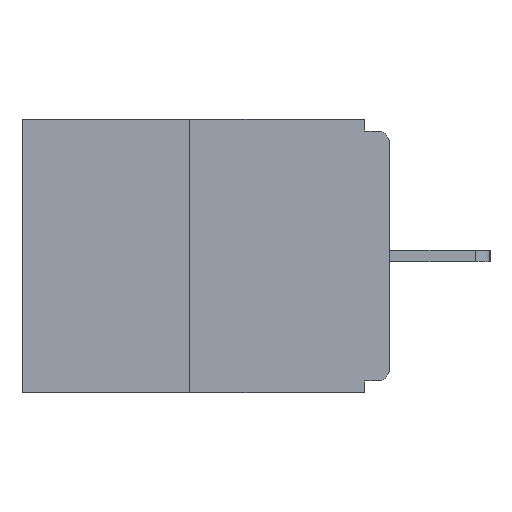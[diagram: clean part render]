
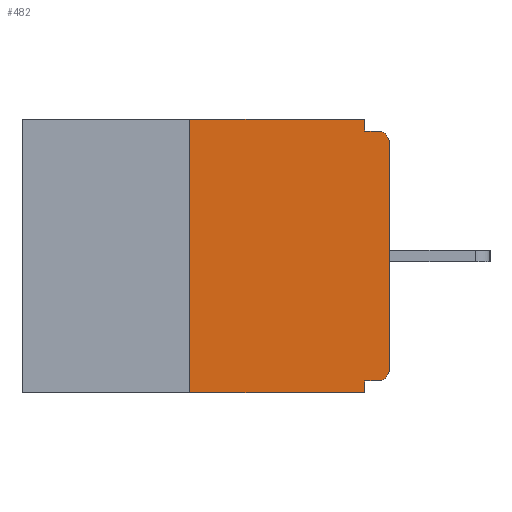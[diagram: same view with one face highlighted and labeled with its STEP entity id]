
A CAD part, left-side view. The second image highlights one B-rep face of the part: STEP entity #482.
In plain terms, the highlighted planar face has unit normal (-1, 0, 0).
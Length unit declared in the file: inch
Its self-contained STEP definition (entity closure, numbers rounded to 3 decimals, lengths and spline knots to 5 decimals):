
#51 = ORIENTED_EDGE ( 'NONE', *, *, #4367, .T. ) ;
#288 = DIRECTION ( 'NONE',  ( 0., 0., 1. ) ) ;
#311 = DIRECTION ( 'NONE',  ( -1., 0., 0. ) ) ;
#482 = ADVANCED_FACE ( 'NONE', ( #3917 ), #5129, .F. ) ;
#664 = AXIS2_PLACEMENT_3D ( 'NONE', #2507, #10840, #3674 ) ;
#820 = VERTEX_POINT ( 'NONE', #11308 ) ;
#857 = EDGE_CURVE ( 'NONE', #13726, #4578, #2613, .T. ) ;
#947 = VERTEX_POINT ( 'NONE', #15404 ) ;
#965 = EDGE_CURVE ( 'NONE', #13865, #2739, #7038, .T. ) ;
#1092 = AXIS2_PLACEMENT_3D ( 'NONE', #5073, #3951, #8962 ) ;
#1094 = VECTOR ( 'NONE', #6309, 39.37008 ) ;
#1556 = CARTESIAN_POINT ( 'NONE',  ( 0., 0., -0.328 ) ) ;
#1710 = EDGE_CURVE ( 'NONE', #14695, #947, #11724, .T. ) ;
#1881 = ORIENTED_EDGE ( 'NONE', *, *, #857, .T. ) ;
#1944 = ORIENTED_EDGE ( 'NONE', *, *, #12583, .F. ) ;
#2138 = DIRECTION ( 'NONE',  ( 0., 0., -1. ) ) ;
#2236 = VECTOR ( 'NONE', #12842, 39.37008 ) ;
#2246 = LINE ( 'NONE', #11869, #4642 ) ;
#2437 = CARTESIAN_POINT ( 'NONE',  ( 0., 0.031, -0.343 ) ) ;
#2507 = CARTESIAN_POINT ( 'NONE',  ( 0., 0.015, -0.313 ) ) ;
#2613 = LINE ( 'NONE', #5681, #2236 ) ;
#2739 = VERTEX_POINT ( 'NONE', #4199 ) ;
#3428 = VECTOR ( 'NONE', #14639, 39.37008 ) ;
#3674 = DIRECTION ( 'NONE',  ( 0., 0., -1. ) ) ;
#3846 = CARTESIAN_POINT ( 'NONE',  ( 0., 0.25, 0. ) ) ;
#3917 = FACE_OUTER_BOUND ( 'NONE', #11331, .T. ) ;
#3951 = DIRECTION ( 'NONE',  ( 1., 0., 0. ) ) ;
#4199 = CARTESIAN_POINT ( 'NONE',  ( 0., 0.031, -0.343 ) ) ;
#4367 = EDGE_CURVE ( 'NONE', #8705, #2739, #2246, .T. ) ;
#4440 = VECTOR ( 'NONE', #14059, 39.37008 ) ;
#4485 = CARTESIAN_POINT ( 'NONE',  ( 0., 0., -0.015 ) ) ;
#4578 = VERTEX_POINT ( 'NONE', #5940 ) ;
#4642 = VECTOR ( 'NONE', #11349, 39.37008 ) ;
#4662 = AXIS2_PLACEMENT_3D ( 'NONE', #7464, #311, #8691 ) ;
#5073 = CARTESIAN_POINT ( 'NONE',  ( 0., 0.46, 0. ) ) ;
#5129 = PLANE ( 'NONE',  #1092 ) ;
#5216 = ORIENTED_EDGE ( 'NONE', *, *, #12276, .T. ) ;
#5488 = VERTEX_POINT ( 'NONE', #15038 ) ;
#5672 = DIRECTION ( 'NONE',  ( 0., -1., 0. ) ) ;
#5681 = CARTESIAN_POINT ( 'NONE',  ( 0., 0., 0. ) ) ;
#5841 = ORIENTED_EDGE ( 'NONE', *, *, #1710, .F. ) ;
#5864 = ORIENTED_EDGE ( 'NONE', *, *, #10852, .F. ) ;
#5940 = CARTESIAN_POINT ( 'NONE',  ( 0., 0., -0.03 ) ) ;
#6309 = DIRECTION ( 'NONE',  ( 0., 0., -1. ) ) ;
#6573 = ORIENTED_EDGE ( 'NONE', *, *, #15152, .F. ) ;
#7038 = LINE ( 'NONE', #2437, #1094 ) ;
#7068 = CARTESIAN_POINT ( 'NONE',  ( 0., 0.015, -0.015 ) ) ;
#7464 = CARTESIAN_POINT ( 'NONE',  ( 0., 0.015, -0.03 ) ) ;
#7613 = LINE ( 'NONE', #15224, #4440 ) ;
#8201 = CIRCLE ( 'NONE', #4662, 0.015 ) ;
#8691 = DIRECTION ( 'NONE',  ( 0., 0., -1. ) ) ;
#8705 = VERTEX_POINT ( 'NONE', #15362 ) ;
#8851 = CARTESIAN_POINT ( 'NONE',  ( 0., 0., -0.313 ) ) ;
#8962 = DIRECTION ( 'NONE',  ( 0., 0., -1. ) ) ;
#9636 = CARTESIAN_POINT ( 'NONE',  ( 0., 0.031, 0. ) ) ;
#9746 = CIRCLE ( 'NONE', #664, 0.015 ) ;
#10840 = DIRECTION ( 'NONE',  ( -1., 0., 0. ) ) ;
#10852 = EDGE_CURVE ( 'NONE', #5488, #13865, #12195, .T. ) ;
#11308 = CARTESIAN_POINT ( 'NONE',  ( 0., 0.25, 0. ) ) ;
#11331 = EDGE_LOOP ( 'NONE', ( #6573, #14446, #51, #13352, #5864, #13366, #1881, #5216, #1944, #5841 ) ) ;
#11349 = DIRECTION ( 'NONE',  ( 0., -1., 0. ) ) ;
#11724 = LINE ( 'NONE', #9636, #14072 ) ;
#11730 = LINE ( 'NONE', #3846, #14150 ) ;
#11869 = CARTESIAN_POINT ( 'NONE',  ( 0., 0.46, -0.343 ) ) ;
#12106 = EDGE_CURVE ( 'NONE', #5488, #13726, #9746, .T. ) ;
#12195 = LINE ( 'NONE', #1556, #3428 ) ;
#12213 = CARTESIAN_POINT ( 'NONE',  ( 0., 0.031, 0. ) ) ;
#12276 = EDGE_CURVE ( 'NONE', #4578, #12749, #8201, .T. ) ;
#12583 = EDGE_CURVE ( 'NONE', #947, #12749, #15267, .T. ) ;
#12633 = CARTESIAN_POINT ( 'NONE',  ( 0., 0.031, -0.328 ) ) ;
#12749 = VERTEX_POINT ( 'NONE', #7068 ) ;
#12842 = DIRECTION ( 'NONE',  ( 0., 0., 1. ) ) ;
#12862 = VECTOR ( 'NONE', #5672, 39.37008 ) ;
#13352 = ORIENTED_EDGE ( 'NONE', *, *, #965, .F. ) ;
#13366 = ORIENTED_EDGE ( 'NONE', *, *, #12106, .T. ) ;
#13497 = EDGE_CURVE ( 'NONE', #8705, #820, #11730, .T. ) ;
#13726 = VERTEX_POINT ( 'NONE', #8851 ) ;
#13865 = VERTEX_POINT ( 'NONE', #12633 ) ;
#14059 = DIRECTION ( 'NONE',  ( 0., -1., 0. ) ) ;
#14072 = VECTOR ( 'NONE', #2138, 39.37008 ) ;
#14150 = VECTOR ( 'NONE', #288, 39.37008 ) ;
#14446 = ORIENTED_EDGE ( 'NONE', *, *, #13497, .F. ) ;
#14639 = DIRECTION ( 'NONE',  ( 0., 1., 0. ) ) ;
#14695 = VERTEX_POINT ( 'NONE', #12213 ) ;
#15038 = CARTESIAN_POINT ( 'NONE',  ( 0., 0.015, -0.328 ) ) ;
#15152 = EDGE_CURVE ( 'NONE', #820, #14695, #7613, .T. ) ;
#15224 = CARTESIAN_POINT ( 'NONE',  ( 0., 0.46, 0. ) ) ;
#15267 = LINE ( 'NONE', #4485, #12862 ) ;
#15362 = CARTESIAN_POINT ( 'NONE',  ( 0., 0.25, -0.343 ) ) ;
#15404 = CARTESIAN_POINT ( 'NONE',  ( 0., 0.031, -0.015 ) ) ;
